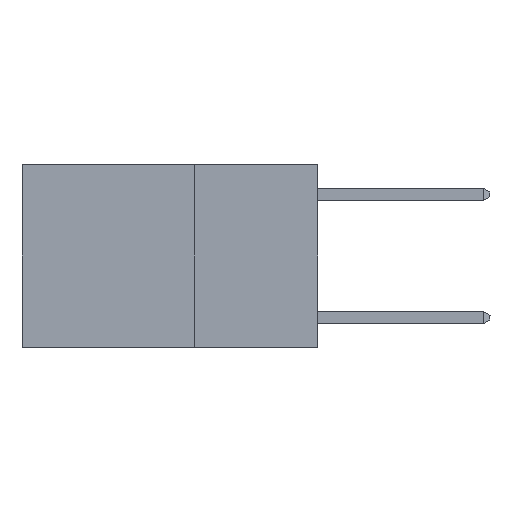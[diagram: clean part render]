
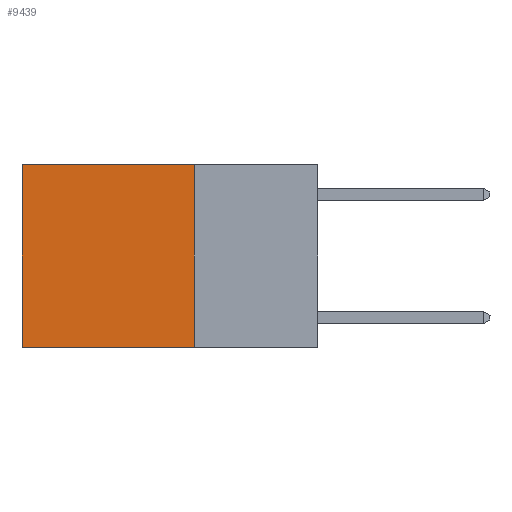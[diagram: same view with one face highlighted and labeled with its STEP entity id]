
A CAD part, left-side view. The second image highlights one B-rep face of the part: STEP entity #9439.
In plain terms, the highlighted planar face has unit normal (-1, 0, 0).
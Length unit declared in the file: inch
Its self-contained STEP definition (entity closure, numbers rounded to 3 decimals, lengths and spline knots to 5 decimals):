
#585 = ORIENTED_EDGE ( 'NONE', *, *, #6420, .F. ) ;
#1276 = CARTESIAN_POINT ( 'NONE',  ( 0.2625, 0.6, 0. ) ) ;
#1348 = DIRECTION ( 'NONE',  ( 0., 1., 0. ) ) ;
#1981 = EDGE_CURVE ( 'NONE', #24774, #16327, #8580, .T. ) ;
#1989 = DIRECTION ( 'NONE',  ( 0., 0., -1. ) ) ;
#3655 = CARTESIAN_POINT ( 'NONE',  ( 0.2625, 0.25, 0. ) ) ;
#4050 = LINE ( 'NONE', #19869, #9200 ) ;
#4236 = VERTEX_POINT ( 'NONE', #26325 ) ;
#4262 = ORIENTED_EDGE ( 'NONE', *, *, #1981, .T. ) ;
#4629 = DIRECTION ( 'NONE',  ( 0., 0., -1. ) ) ;
#5930 = VECTOR ( 'NONE', #27521, 39.37008 ) ;
#6420 = EDGE_CURVE ( 'NONE', #24774, #27914, #7298, .T. ) ;
#7264 = DIRECTION ( 'NONE',  ( 0., 1., 0. ) ) ;
#7298 = LINE ( 'NONE', #3655, #5930 ) ;
#8101 = FACE_OUTER_BOUND ( 'NONE', #11698, .T. ) ;
#8132 = CARTESIAN_POINT ( 'NONE',  ( 0.2625, 0.25, -0.37 ) ) ;
#8549 = PLANE ( 'NONE',  #15521 ) ;
#8580 = LINE ( 'NONE', #23207, #25157 ) ;
#9200 = VECTOR ( 'NONE', #4629, 39.37008 ) ;
#9439 = ADVANCED_FACE ( 'NONE', ( #8101 ), #8549, .F. ) ;
#9865 = CARTESIAN_POINT ( 'NONE',  ( 0.2625, 0.25, 0. ) ) ;
#11698 = EDGE_LOOP ( 'NONE', ( #18534, #19113, #585, #4262 ) ) ;
#15090 = DIRECTION ( 'NONE',  ( 1., 0., 0. ) ) ;
#15481 = LINE ( 'NONE', #15908, #26272 ) ;
#15521 = AXIS2_PLACEMENT_3D ( 'NONE', #27954, #15090, #1989 ) ;
#15908 = CARTESIAN_POINT ( 'NONE',  ( 0.2625, 0.25, -0.37 ) ) ;
#16327 = VERTEX_POINT ( 'NONE', #1276 ) ;
#18534 = ORIENTED_EDGE ( 'NONE', *, *, #26855, .T. ) ;
#19113 = ORIENTED_EDGE ( 'NONE', *, *, #27642, .F. ) ;
#19869 = CARTESIAN_POINT ( 'NONE',  ( 0.2625, 0.6, 0. ) ) ;
#23207 = CARTESIAN_POINT ( 'NONE',  ( 0.2625, 0.25, 0. ) ) ;
#24774 = VERTEX_POINT ( 'NONE', #9865 ) ;
#25157 = VECTOR ( 'NONE', #1348, 39.37008 ) ;
#26272 = VECTOR ( 'NONE', #7264, 39.37008 ) ;
#26325 = CARTESIAN_POINT ( 'NONE',  ( 0.2625, 0.6, -0.37 ) ) ;
#26855 = EDGE_CURVE ( 'NONE', #16327, #4236, #4050, .T. ) ;
#27521 = DIRECTION ( 'NONE',  ( 0., 0., -1. ) ) ;
#27642 = EDGE_CURVE ( 'NONE', #27914, #4236, #15481, .T. ) ;
#27914 = VERTEX_POINT ( 'NONE', #8132 ) ;
#27954 = CARTESIAN_POINT ( 'NONE',  ( 0.2625, 0.25, 0. ) ) ;
